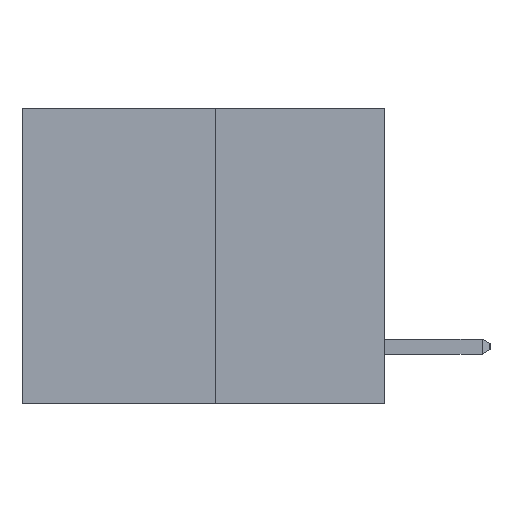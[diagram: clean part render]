
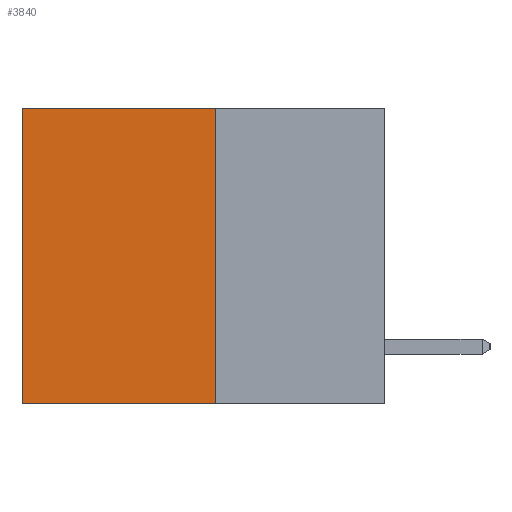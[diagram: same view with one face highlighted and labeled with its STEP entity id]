
A CAD part, left-side view. The second image highlights one B-rep face of the part: STEP entity #3840.
In plain terms, the highlighted planar face has unit normal (-1, 0, 0).
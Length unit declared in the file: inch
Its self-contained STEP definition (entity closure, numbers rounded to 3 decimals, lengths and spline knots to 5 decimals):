
#553 = EDGE_CURVE ( 'NONE', #15489, #4176, #1601, .T. ) ;
#1601 = LINE ( 'NONE', #9663, #7498 ) ;
#1987 = CARTESIAN_POINT ( 'NONE',  ( 0.3165, 0.28, -0.49 ) ) ;
#2343 = CARTESIAN_POINT ( 'NONE',  ( 0.3165, 0.28, -0.49 ) ) ;
#2711 = LINE ( 'NONE', #6789, #19947 ) ;
#3840 = ADVANCED_FACE ( 'NONE', ( #20790 ), #16998, .F. ) ;
#4176 = VERTEX_POINT ( 'NONE', #13397 ) ;
#4568 = EDGE_CURVE ( 'NONE', #12887, #18993, #2711, .T. ) ;
#5549 = EDGE_CURVE ( 'NONE', #4176, #18993, #15842, .T. ) ;
#6624 = ORIENTED_EDGE ( 'NONE', *, *, #9147, .F. ) ;
#6789 = CARTESIAN_POINT ( 'NONE',  ( 0.3165, 0.28, -0.49 ) ) ;
#7498 = VECTOR ( 'NONE', #22363, 39.37008 ) ;
#8167 = ORIENTED_EDGE ( 'NONE', *, *, #553, .T. ) ;
#9100 = VECTOR ( 'NONE', #13223, 39.37008 ) ;
#9147 = EDGE_CURVE ( 'NONE', #15489, #12887, #11649, .T. ) ;
#9663 = CARTESIAN_POINT ( 'NONE',  ( 0.3165, 0.28, 0. ) ) ;
#9699 = DIRECTION ( 'NONE',  ( 0., 0., -1. ) ) ;
#10338 = CARTESIAN_POINT ( 'NONE',  ( 0.3165, 0.6, -0.49 ) ) ;
#10500 = DIRECTION ( 'NONE',  ( 0., 0., -1. ) ) ;
#10807 = CARTESIAN_POINT ( 'NONE',  ( 0.3165, 0.28, 0. ) ) ;
#11649 = LINE ( 'NONE', #18858, #9100 ) ;
#12084 = EDGE_LOOP ( 'NONE', ( #17774, #22219, #6624, #8167 ) ) ;
#12637 = CARTESIAN_POINT ( 'NONE',  ( 0.3165, 0.6, -0.49 ) ) ;
#12887 = VERTEX_POINT ( 'NONE', #1987 ) ;
#13223 = DIRECTION ( 'NONE',  ( 0., 0., -1. ) ) ;
#13397 = CARTESIAN_POINT ( 'NONE',  ( 0.3165, 0.6, 0. ) ) ;
#14945 = DIRECTION ( 'NONE',  ( 1., 0., 0. ) ) ;
#15489 = VERTEX_POINT ( 'NONE', #10807 ) ;
#15842 = LINE ( 'NONE', #10338, #17826 ) ;
#16998 = PLANE ( 'NONE',  #18948 ) ;
#17290 = DIRECTION ( 'NONE',  ( 0., 1., 0. ) ) ;
#17774 = ORIENTED_EDGE ( 'NONE', *, *, #5549, .T. ) ;
#17826 = VECTOR ( 'NONE', #10500, 39.37008 ) ;
#18858 = CARTESIAN_POINT ( 'NONE',  ( 0.3165, 0.28, -0.49 ) ) ;
#18948 = AXIS2_PLACEMENT_3D ( 'NONE', #2343, #14945, #9699 ) ;
#18993 = VERTEX_POINT ( 'NONE', #12637 ) ;
#19947 = VECTOR ( 'NONE', #17290, 39.37008 ) ;
#20790 = FACE_OUTER_BOUND ( 'NONE', #12084, .T. ) ;
#22219 = ORIENTED_EDGE ( 'NONE', *, *, #4568, .F. ) ;
#22363 = DIRECTION ( 'NONE',  ( 0., 1., 0. ) ) ;
